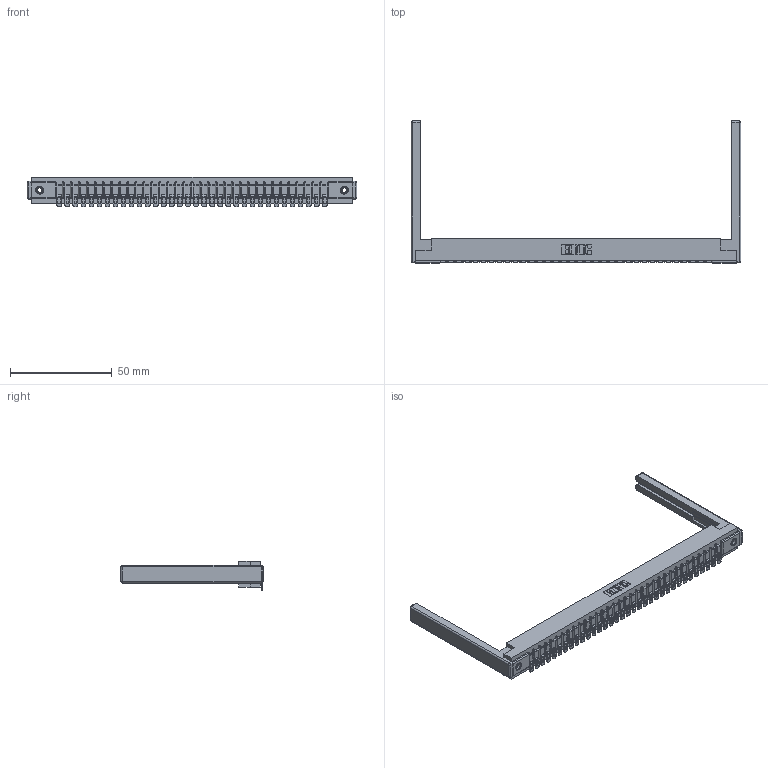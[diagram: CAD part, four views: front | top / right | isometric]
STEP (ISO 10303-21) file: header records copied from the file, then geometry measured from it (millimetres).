
FILE_DESCRIPTION (( 'STEP AP203' ), '1' );
FILE_NAME ('357-034-454-168.STEP', '2020-10-02T11:07:37', ( '' ), ( '' ), 'SwSTEP 2.0', 'SolidWorks 2020', '' );
FILE_SCHEMA (( 'CONFIG_CONTROL_DESIGN' ));
Length unit declared in the file: inch
Products named in the file (5): 345-250-001_345-250-001-102; 357-034-454-168; 307-290-002_554; 307 Part_.156 Dia Mounting Holes; 307-220-068
Assembly tree (39 placements, depth 2):
  357-034-454-168
    307 Part_.156 Dia Mounting Holes
    307-290-002_554  x34
    307-220-068  x2
    345-250-001_345-250-001-102  x2
Bounding box: 162.15 x 69.98 x 14.52 mm (x, y, z)
Volume: 21682.7 mm3; surface area: 25675.6 mm2
Topology: 39 solids, 39 shells, 3061 faces, 9315 edges, 6094 vertices
Faces by surface type: plane 1722, cylinder 1245, sphere 78, cone 12, torus 4
Entity records: 33858 total; most frequent: CARTESIAN_POINT 5675, ORIENTED_EDGE 5654, DIRECTION 5541, EDGE_CURVE 2827, LINE 2153, VECTOR 2153, VERTEX_POINT 1828, AXIS2_PLACEMENT_3D 1694
